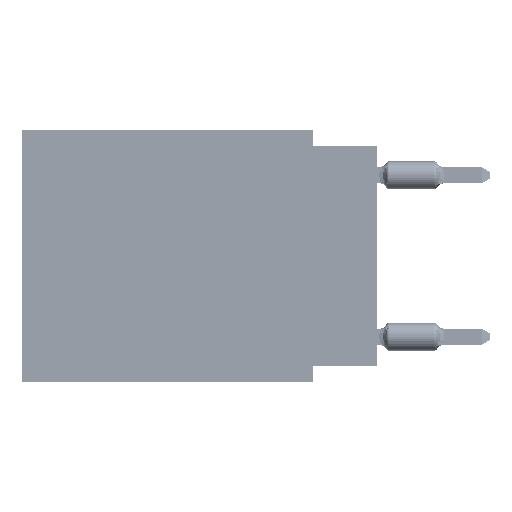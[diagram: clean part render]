
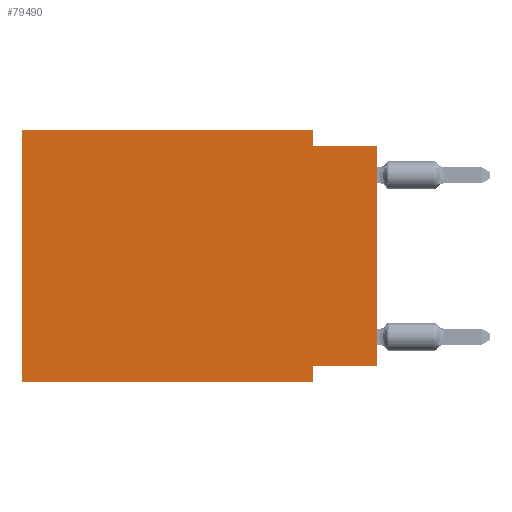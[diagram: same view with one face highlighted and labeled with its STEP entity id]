
A CAD part, left-side view. The second image highlights one B-rep face of the part: STEP entity #79490.
In plain terms, the highlighted planar face has unit normal (-1, 0, 0).
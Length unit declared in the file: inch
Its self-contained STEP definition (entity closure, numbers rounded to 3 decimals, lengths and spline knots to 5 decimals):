
#1216 = CARTESIAN_POINT ( 'NONE',  ( 0., 0.55, 0. ) ) ;
#1647 = DIRECTION ( 'NONE',  ( 0., 0., -1. ) ) ;
#3088 = VERTEX_POINT ( 'NONE', #77229 ) ;
#7230 = VECTOR ( 'NONE', #53721, 39.37008 ) ;
#12622 = CARTESIAN_POINT ( 'NONE',  ( 0., 0., -0.025 ) ) ;
#12675 = CARTESIAN_POINT ( 'NONE',  ( 0., 0., -0.365 ) ) ;
#13163 = DIRECTION ( 'NONE',  ( 0., -1., 0. ) ) ;
#14705 = LINE ( 'NONE', #68590, #47047 ) ;
#16991 = LINE ( 'NONE', #77505, #25218 ) ;
#17824 = ORIENTED_EDGE ( 'NONE', *, *, #41407, .F. ) ;
#21711 = VECTOR ( 'NONE', #62158, 39.37008 ) ;
#22076 = CARTESIAN_POINT ( 'NONE',  ( 0., 0.55, -0.39 ) ) ;
#23277 = EDGE_CURVE ( 'NONE', #38724, #30283, #14705, .T. ) ;
#25218 = VECTOR ( 'NONE', #50557, 39.37008 ) ;
#26430 = VERTEX_POINT ( 'NONE', #54799 ) ;
#26987 = VERTEX_POINT ( 'NONE', #37432 ) ;
#27939 = VECTOR ( 'NONE', #53534, 39.37008 ) ;
#30283 = VERTEX_POINT ( 'NONE', #55221 ) ;
#33029 = CARTESIAN_POINT ( 'NONE',  ( 0., 0.55, -0.39 ) ) ;
#34139 = ORIENTED_EDGE ( 'NONE', *, *, #23277, .F. ) ;
#34750 = FACE_OUTER_BOUND ( 'NONE', #62002, .T. ) ;
#35849 = ORIENTED_EDGE ( 'NONE', *, *, #70069, .F. ) ;
#37432 = CARTESIAN_POINT ( 'NONE',  ( 0., 0., -0.025 ) ) ;
#38724 = VERTEX_POINT ( 'NONE', #75323 ) ;
#39838 = LINE ( 'NONE', #79166, #27939 ) ;
#40215 = ORIENTED_EDGE ( 'NONE', *, *, #85422, .T. ) ;
#40396 = DIRECTION ( 'NONE',  ( 0., 0., 1. ) ) ;
#40483 = LINE ( 'NONE', #12675, #7230 ) ;
#40948 = CARTESIAN_POINT ( 'NONE',  ( 0., 0.55, 0. ) ) ;
#41407 = EDGE_CURVE ( 'NONE', #26430, #3088, #40483, .T. ) ;
#41687 = VECTOR ( 'NONE', #66919, 39.37008 ) ;
#47047 = VECTOR ( 'NONE', #82694, 39.37008 ) ;
#47503 = ORIENTED_EDGE ( 'NONE', *, *, #82341, .T. ) ;
#47920 = VECTOR ( 'NONE', #40396, 39.37008 ) ;
#48171 = EDGE_CURVE ( 'NONE', #3088, #64818, #16991, .T. ) ;
#50557 = DIRECTION ( 'NONE',  ( 0., 0., -1. ) ) ;
#51758 = AXIS2_PLACEMENT_3D ( 'NONE', #1216, #68755, #1647 ) ;
#53534 = DIRECTION ( 'NONE',  ( 0., 0., 1. ) ) ;
#53721 = DIRECTION ( 'NONE',  ( 0., 1., 0. ) ) ;
#53905 = ORIENTED_EDGE ( 'NONE', *, *, #72725, .F. ) ;
#54799 = CARTESIAN_POINT ( 'NONE',  ( 0., 0., -0.365 ) ) ;
#55221 = CARTESIAN_POINT ( 'NONE',  ( 0., 0.1, -0.025 ) ) ;
#56073 = EDGE_CURVE ( 'NONE', #63425, #38724, #62590, .T. ) ;
#59516 = VECTOR ( 'NONE', #13163, 39.37008 ) ;
#60308 = LINE ( 'NONE', #12622, #41687 ) ;
#61681 = PLANE ( 'NONE',  #51758 ) ;
#62002 = EDGE_LOOP ( 'NONE', ( #47503, #35849, #34139, #74986, #53905, #40215, #64767, #17824 ) ) ;
#62158 = DIRECTION ( 'NONE',  ( 0., -1., 0. ) ) ;
#62590 = LINE ( 'NONE', #81163, #21711 ) ;
#63425 = VERTEX_POINT ( 'NONE', #40948 ) ;
#64767 = ORIENTED_EDGE ( 'NONE', *, *, #48171, .F. ) ;
#64818 = VERTEX_POINT ( 'NONE', #87217 ) ;
#66455 = LINE ( 'NONE', #83375, #47920 ) ;
#66919 = DIRECTION ( 'NONE',  ( 0., -1., 0. ) ) ;
#68590 = CARTESIAN_POINT ( 'NONE',  ( 0., 0.1, 0. ) ) ;
#68755 = DIRECTION ( 'NONE',  ( 1., 0., 0. ) ) ;
#70069 = EDGE_CURVE ( 'NONE', #30283, #26987, #60308, .T. ) ;
#71945 = LINE ( 'NONE', #33029, #59516 ) ;
#72725 = EDGE_CURVE ( 'NONE', #86958, #63425, #39838, .T. ) ;
#74986 = ORIENTED_EDGE ( 'NONE', *, *, #56073, .F. ) ;
#75323 = CARTESIAN_POINT ( 'NONE',  ( 0., 0.1, 0. ) ) ;
#77229 = CARTESIAN_POINT ( 'NONE',  ( 0., 0.1, -0.365 ) ) ;
#77505 = CARTESIAN_POINT ( 'NONE',  ( 0., 0.1, -0.39 ) ) ;
#79166 = CARTESIAN_POINT ( 'NONE',  ( 0., 0.55, 0. ) ) ;
#79490 = ADVANCED_FACE ( 'NONE', ( #34750 ), #61681, .F. ) ;
#81163 = CARTESIAN_POINT ( 'NONE',  ( 0., 0.55, 0. ) ) ;
#82341 = EDGE_CURVE ( 'NONE', #26430, #26987, #66455, .T. ) ;
#82694 = DIRECTION ( 'NONE',  ( 0., 0., -1. ) ) ;
#83375 = CARTESIAN_POINT ( 'NONE',  ( 0., 0., 0. ) ) ;
#85422 = EDGE_CURVE ( 'NONE', #86958, #64818, #71945, .T. ) ;
#86958 = VERTEX_POINT ( 'NONE', #22076 ) ;
#87217 = CARTESIAN_POINT ( 'NONE',  ( 0., 0.1, -0.39 ) ) ;
